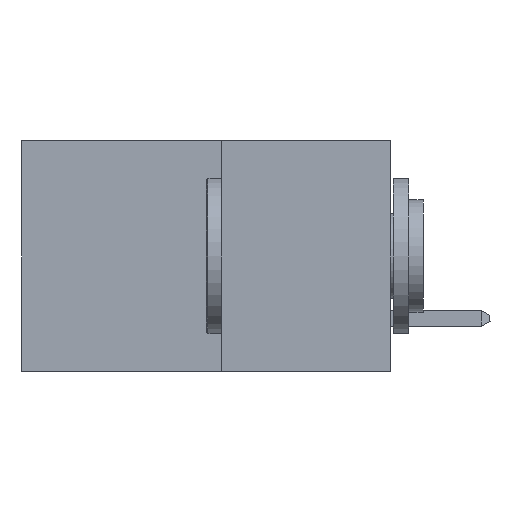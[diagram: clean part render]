
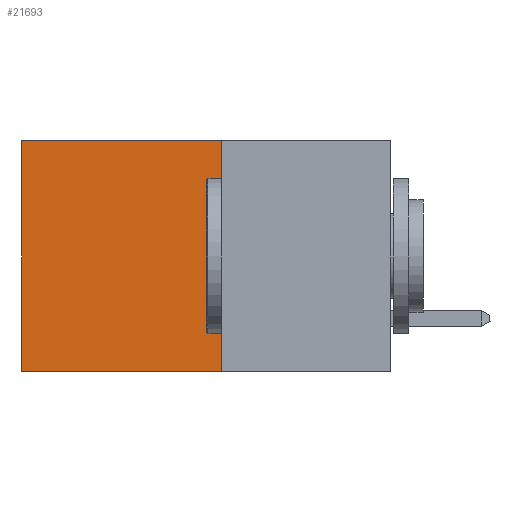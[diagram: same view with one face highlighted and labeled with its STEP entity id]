
A CAD part, left-side view. The second image highlights one B-rep face of the part: STEP entity #21693.
In plain terms, the highlighted planar face has unit normal (-1, 0, 0).
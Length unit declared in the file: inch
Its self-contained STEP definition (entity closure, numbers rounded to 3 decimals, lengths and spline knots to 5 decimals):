
#1857 = EDGE_CURVE ( 'NONE', #5820, #23064, #18044, .T. ) ;
#2072 = CARTESIAN_POINT ( 'NONE',  ( 0.277, 0.27, -0.37 ) ) ;
#2460 = CARTESIAN_POINT ( 'NONE',  ( 0.277, 0.27, 0. ) ) ;
#4778 = VERTEX_POINT ( 'NONE', #15790 ) ;
#5820 = VERTEX_POINT ( 'NONE', #7077 ) ;
#7077 = CARTESIAN_POINT ( 'NONE',  ( 0.277, 0.59, 0. ) ) ;
#7719 = EDGE_CURVE ( 'NONE', #9343, #23064, #32877, .T. ) ;
#8533 = ORIENTED_EDGE ( 'NONE', *, *, #16626, .T. ) ;
#9343 = VERTEX_POINT ( 'NONE', #21901 ) ;
#10260 = VECTOR ( 'NONE', #24647, 39.37008 ) ;
#10631 = CARTESIAN_POINT ( 'NONE',  ( 0.277, 0.27, -0.37 ) ) ;
#10786 = DIRECTION ( 'NONE',  ( 1., 0., 0. ) ) ;
#11605 = EDGE_CURVE ( 'NONE', #4778, #9343, #21785, .T. ) ;
#12541 = ORIENTED_EDGE ( 'NONE', *, *, #7719, .F. ) ;
#12723 = ORIENTED_EDGE ( 'NONE', *, *, #11605, .F. ) ;
#13694 = ORIENTED_EDGE ( 'NONE', *, *, #1857, .T. ) ;
#15790 = CARTESIAN_POINT ( 'NONE',  ( 0.277, 0.27, 0. ) ) ;
#16496 = VECTOR ( 'NONE', #28888, 39.37008 ) ;
#16626 = EDGE_CURVE ( 'NONE', #4778, #5820, #26035, .T. ) ;
#18044 = LINE ( 'NONE', #31886, #10260 ) ;
#19107 = VECTOR ( 'NONE', #23514, 39.37008 ) ;
#19372 = EDGE_LOOP ( 'NONE', ( #13694, #12541, #12723, #8533 ) ) ;
#20511 = DIRECTION ( 'NONE',  ( 0., 1., 0. ) ) ;
#20822 = FACE_OUTER_BOUND ( 'NONE', #19372, .T. ) ;
#21693 = ADVANCED_FACE ( 'NONE', ( #20822 ), #28940, .F. ) ;
#21785 = LINE ( 'NONE', #10631, #16496 ) ;
#21901 = CARTESIAN_POINT ( 'NONE',  ( 0.277, 0.27, -0.37 ) ) ;
#23064 = VERTEX_POINT ( 'NONE', #33217 ) ;
#23514 = DIRECTION ( 'NONE',  ( 0., 1., 0. ) ) ;
#24647 = DIRECTION ( 'NONE',  ( 0., 0., -1. ) ) ;
#26035 = LINE ( 'NONE', #2460, #19107 ) ;
#26427 = CARTESIAN_POINT ( 'NONE',  ( 0.277, 0.27, -0.37 ) ) ;
#26776 = AXIS2_PLACEMENT_3D ( 'NONE', #26427, #10786, #29063 ) ;
#26797 = VECTOR ( 'NONE', #20511, 39.37008 ) ;
#28888 = DIRECTION ( 'NONE',  ( 0., 0., -1. ) ) ;
#28940 = PLANE ( 'NONE',  #26776 ) ;
#29063 = DIRECTION ( 'NONE',  ( 0., 0., -1. ) ) ;
#31886 = CARTESIAN_POINT ( 'NONE',  ( 0.277, 0.59, -0.37 ) ) ;
#32877 = LINE ( 'NONE', #2072, #26797 ) ;
#33217 = CARTESIAN_POINT ( 'NONE',  ( 0.277, 0.59, -0.37 ) ) ;
